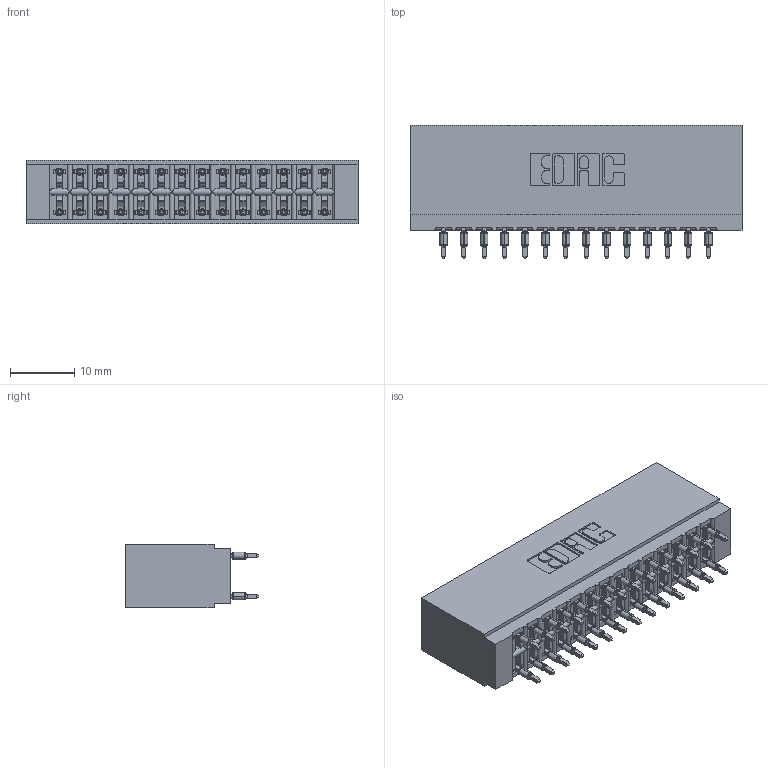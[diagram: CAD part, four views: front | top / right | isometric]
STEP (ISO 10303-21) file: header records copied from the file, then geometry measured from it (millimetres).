
FILE_DESCRIPTION (( 'STEP AP203' ), '1' );
FILE_NAME ('746-028-560-201.STEP', '2026-02-26T23:38:27', ( '' ), ( '' ), 'SwSTEP 2.0', 'SolidWorks 2023', '' );
FILE_SCHEMA (( 'CONFIG_CONTROL_DESIGN' ));
Length unit declared in the file: millimetre
Products named in the file (3): 746 Part_.515 Slot Depth - 01; 746-292-001_560; 746-028-560-201
Assembly tree (29 placements, depth 2):
  746-028-560-201
    746 Part_.515 Slot Depth - 01
    746-292-001_560  x28
Bounding box: 51.69 x 20.82 x 9.91 mm (x, y, z)
Volume: 5817.8 mm3; surface area: 9236.9 mm2
Topology: 29 solids, 29 shells, 2743 faces, 7627 edges, 4893 vertices
Faces by surface type: plane 1371, cylinder 644, bspline 560, torus 168
Entity records: 25744 total; most frequent: CARTESIAN_POINT 5359, ORIENTED_EDGE 4346, DIRECTION 3683, EDGE_CURVE 2173, LINE 1841, VECTOR 1841, VERTEX_POINT 1437, AXIS2_PLACEMENT_3D 921
